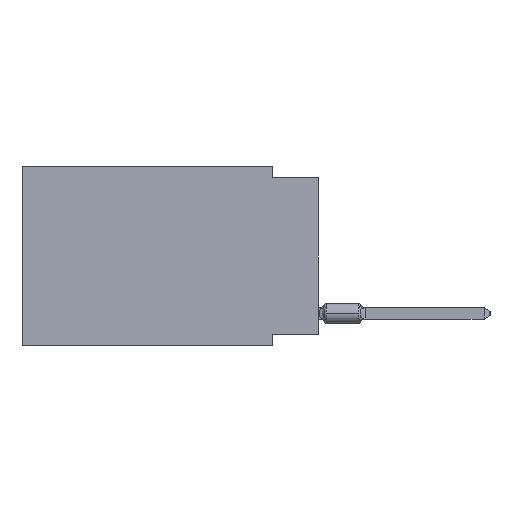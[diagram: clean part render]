
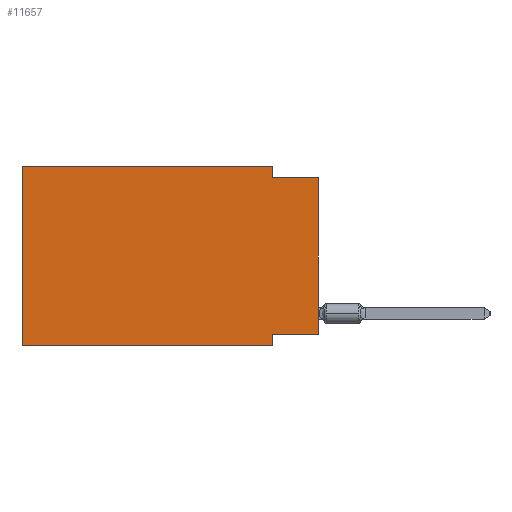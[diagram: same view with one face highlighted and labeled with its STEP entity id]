
A CAD part, left-side view. The second image highlights one B-rep face of the part: STEP entity #11657.
In plain terms, the highlighted planar face has unit normal (-1, 0, 0).
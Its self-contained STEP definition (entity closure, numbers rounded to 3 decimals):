
#1575 = ORIENTED_EDGE ( 'NONE', *, *, #7435, .F. ) ;
#1765 = CARTESIAN_POINT ( 'NONE',  ( 0., 2.54, -9.906 ) ) ;
#1914 = VERTEX_POINT ( 'NONE', #66476 ) ;
#2816 = CARTESIAN_POINT ( 'NONE',  ( 0., 2.54, -0.635 ) ) ;
#3316 = AXIS2_PLACEMENT_3D ( 'NONE', #41360, #73865, #26940 ) ;
#5904 = ORIENTED_EDGE ( 'NONE', *, *, #52467, .T. ) ;
#6120 = VERTEX_POINT ( 'NONE', #1765 ) ;
#6812 = VECTOR ( 'NONE', #83043, 1000. ) ;
#7435 = EDGE_CURVE ( 'NONE', #46336, #26216, #16249, .T. ) ;
#8538 = DIRECTION ( 'NONE',  ( 0., 0., -1. ) ) ;
#9066 = CARTESIAN_POINT ( 'NONE',  ( 0., 2.54, 0. ) ) ;
#10237 = LINE ( 'NONE', #56256, #6812 ) ;
#11209 = EDGE_CURVE ( 'NONE', #21109, #15124, #45470, .T. ) ;
#11657 = ADVANCED_FACE ( 'NONE', ( #27361 ), #80875, .F. ) ;
#15124 = VERTEX_POINT ( 'NONE', #60355 ) ;
#16249 = LINE ( 'NONE', #56127, #38071 ) ;
#16537 = DIRECTION ( 'NONE',  ( 0., 0., -1. ) ) ;
#20528 = CARTESIAN_POINT ( 'NONE',  ( 0., 0., -9.271 ) ) ;
#21109 = VERTEX_POINT ( 'NONE', #2816 ) ;
#22728 = VECTOR ( 'NONE', #16537, 1000. ) ;
#25347 = ORIENTED_EDGE ( 'NONE', *, *, #31415, .F. ) ;
#26216 = VERTEX_POINT ( 'NONE', #50183 ) ;
#26940 = DIRECTION ( 'NONE',  ( 0., 0., -1. ) ) ;
#27361 = FACE_OUTER_BOUND ( 'NONE', #55192, .T. ) ;
#29581 = LINE ( 'NONE', #30015, #37225 ) ;
#30015 = CARTESIAN_POINT ( 'NONE',  ( 0., 2.54, -9.906 ) ) ;
#31415 = EDGE_CURVE ( 'NONE', #33543, #46336, #79781, .T. ) ;
#33543 = VERTEX_POINT ( 'NONE', #67716 ) ;
#37225 = VECTOR ( 'NONE', #8538, 1000. ) ;
#38071 = VECTOR ( 'NONE', #84199, 1000. ) ;
#39759 = CARTESIAN_POINT ( 'NONE',  ( 0., 0., -0.635 ) ) ;
#41115 = DIRECTION ( 'NONE',  ( 0., 0., 1. ) ) ;
#41360 = CARTESIAN_POINT ( 'NONE',  ( 0., 16.383, 0. ) ) ;
#42814 = LINE ( 'NONE', #9066, #22728 ) ;
#45470 = LINE ( 'NONE', #39759, #63535 ) ;
#46336 = VERTEX_POINT ( 'NONE', #55245 ) ;
#47245 = DIRECTION ( 'NONE',  ( 0., 1., 0. ) ) ;
#48112 = DIRECTION ( 'NONE',  ( 0., -1., 0. ) ) ;
#49946 = VECTOR ( 'NONE', #41115, 1000. ) ;
#50183 = CARTESIAN_POINT ( 'NONE',  ( 0., 2.54, 0. ) ) ;
#52467 = EDGE_CURVE ( 'NONE', #33543, #6120, #73609, .T. ) ;
#53161 = EDGE_CURVE ( 'NONE', #1914, #76516, #85903, .T. ) ;
#55192 = EDGE_LOOP ( 'NONE', ( #61038, #59195, #56481, #1575, #25347, #5904, #86717, #70090 ) ) ;
#55245 = CARTESIAN_POINT ( 'NONE',  ( 0., 16.383, 0. ) ) ;
#55595 = CARTESIAN_POINT ( 'NONE',  ( 0., 2.54, -9.271 ) ) ;
#56127 = CARTESIAN_POINT ( 'NONE',  ( 0., 16.383, 0. ) ) ;
#56256 = CARTESIAN_POINT ( 'NONE',  ( 0., 0., 0. ) ) ;
#56481 = ORIENTED_EDGE ( 'NONE', *, *, #65554, .F. ) ;
#59195 = ORIENTED_EDGE ( 'NONE', *, *, #11209, .F. ) ;
#60355 = CARTESIAN_POINT ( 'NONE',  ( 0., 0., -0.635 ) ) ;
#61038 = ORIENTED_EDGE ( 'NONE', *, *, #71548, .T. ) ;
#63535 = VECTOR ( 'NONE', #73103, 1000. ) ;
#65554 = EDGE_CURVE ( 'NONE', #26216, #21109, #42814, .T. ) ;
#66476 = CARTESIAN_POINT ( 'NONE',  ( 0., 0., -9.271 ) ) ;
#67027 = CARTESIAN_POINT ( 'NONE',  ( 0., 16.383, -9.906 ) ) ;
#67066 = EDGE_CURVE ( 'NONE', #76516, #6120, #29581, .T. ) ;
#67716 = CARTESIAN_POINT ( 'NONE',  ( 0., 16.383, -9.906 ) ) ;
#70090 = ORIENTED_EDGE ( 'NONE', *, *, #53161, .F. ) ;
#71548 = EDGE_CURVE ( 'NONE', #1914, #15124, #10237, .T. ) ;
#72455 = VECTOR ( 'NONE', #47245, 1000. ) ;
#73103 = DIRECTION ( 'NONE',  ( 0., -1., 0. ) ) ;
#73609 = LINE ( 'NONE', #67027, #83600 ) ;
#73865 = DIRECTION ( 'NONE',  ( 1., 0., 0. ) ) ;
#74033 = CARTESIAN_POINT ( 'NONE',  ( 0., 16.383, 0. ) ) ;
#76516 = VERTEX_POINT ( 'NONE', #55595 ) ;
#79781 = LINE ( 'NONE', #74033, #49946 ) ;
#80875 = PLANE ( 'NONE',  #3316 ) ;
#83043 = DIRECTION ( 'NONE',  ( 0., 0., 1. ) ) ;
#83600 = VECTOR ( 'NONE', #48112, 1000. ) ;
#84199 = DIRECTION ( 'NONE',  ( 0., -1., 0. ) ) ;
#85903 = LINE ( 'NONE', #20528, #72455 ) ;
#86717 = ORIENTED_EDGE ( 'NONE', *, *, #67066, .F. ) ;
